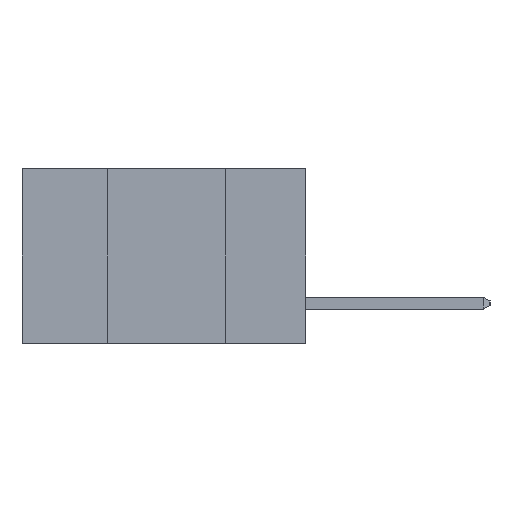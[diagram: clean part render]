
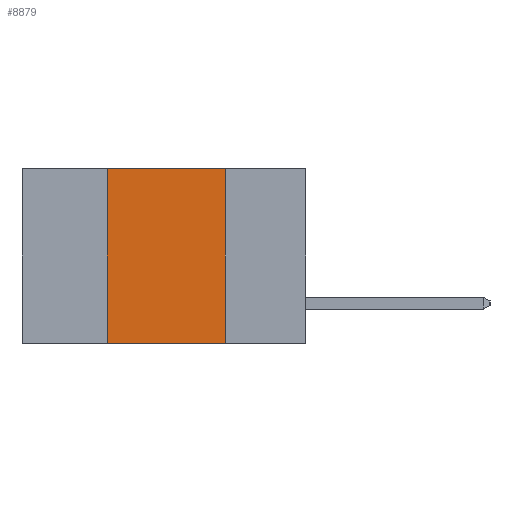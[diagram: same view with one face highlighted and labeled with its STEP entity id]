
A CAD part, left-side view. The second image highlights one B-rep face of the part: STEP entity #8879.
In plain terms, the highlighted planar face has unit normal (-1, 0, 0).
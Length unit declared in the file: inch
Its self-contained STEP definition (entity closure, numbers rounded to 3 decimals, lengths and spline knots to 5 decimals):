
#566 = ORIENTED_EDGE ( 'NONE', *, *, #880, .T. ) ;
#880 = EDGE_CURVE ( 'NONE', #17720, #16504, #20539, .T. ) ;
#1406 = ORIENTED_EDGE ( 'NONE', *, *, #3209, .F. ) ;
#1711 = DIRECTION ( 'NONE',  ( 1., 0., 0. ) ) ;
#1799 = EDGE_CURVE ( 'NONE', #17720, #3957, #25519, .T. ) ;
#2946 = CARTESIAN_POINT ( 'NONE',  ( 0., 0.17, 0. ) ) ;
#3022 = FACE_OUTER_BOUND ( 'NONE', #25710, .T. ) ;
#3209 = EDGE_CURVE ( 'NONE', #24025, #16504, #5426, .T. ) ;
#3957 = VERTEX_POINT ( 'NONE', #11154 ) ;
#4676 = ORIENTED_EDGE ( 'NONE', *, *, #23079, .F. ) ;
#4750 = VECTOR ( 'NONE', #23091, 39.37008 ) ;
#5426 = LINE ( 'NONE', #23874, #4750 ) ;
#6004 = DIRECTION ( 'NONE',  ( 0., 0., 1. ) ) ;
#6144 = VECTOR ( 'NONE', #20796, 39.37008 ) ;
#8879 = ADVANCED_FACE ( 'NONE', ( #3022 ), #25137, .F. ) ;
#10178 = CARTESIAN_POINT ( 'NONE',  ( 0., 0.17, -0.37 ) ) ;
#11154 = CARTESIAN_POINT ( 'NONE',  ( 0., 0.42, 0. ) ) ;
#11302 = CARTESIAN_POINT ( 'NONE',  ( 0., 0.42, 0. ) ) ;
#14728 = CARTESIAN_POINT ( 'NONE',  ( 0., 0.42, -0.37 ) ) ;
#14821 = VECTOR ( 'NONE', #23820, 39.37008 ) ;
#15191 = CARTESIAN_POINT ( 'NONE',  ( 0., 0.6, -0.37 ) ) ;
#15541 = ORIENTED_EDGE ( 'NONE', *, *, #1799, .F. ) ;
#16504 = VERTEX_POINT ( 'NONE', #10178 ) ;
#16593 = DIRECTION ( 'NONE',  ( 0., 0., -1. ) ) ;
#17720 = VERTEX_POINT ( 'NONE', #14728 ) ;
#18652 = CARTESIAN_POINT ( 'NONE',  ( 0., 0.6, 0. ) ) ;
#18658 = CARTESIAN_POINT ( 'NONE',  ( 0., 0.6, 0. ) ) ;
#20486 = VECTOR ( 'NONE', #6004, 39.37008 ) ;
#20539 = LINE ( 'NONE', #15191, #14821 ) ;
#20796 = DIRECTION ( 'NONE',  ( 0., -1., 0. ) ) ;
#21163 = AXIS2_PLACEMENT_3D ( 'NONE', #18652, #1711, #16593 ) ;
#23079 = EDGE_CURVE ( 'NONE', #3957, #24025, #23184, .T. ) ;
#23091 = DIRECTION ( 'NONE',  ( 0., 0., -1. ) ) ;
#23184 = LINE ( 'NONE', #18658, #6144 ) ;
#23820 = DIRECTION ( 'NONE',  ( 0., -1., 0. ) ) ;
#23874 = CARTESIAN_POINT ( 'NONE',  ( 0., 0.17, 0. ) ) ;
#24025 = VERTEX_POINT ( 'NONE', #2946 ) ;
#25137 = PLANE ( 'NONE',  #21163 ) ;
#25519 = LINE ( 'NONE', #11302, #20486 ) ;
#25710 = EDGE_LOOP ( 'NONE', ( #1406, #4676, #15541, #566 ) ) ;
